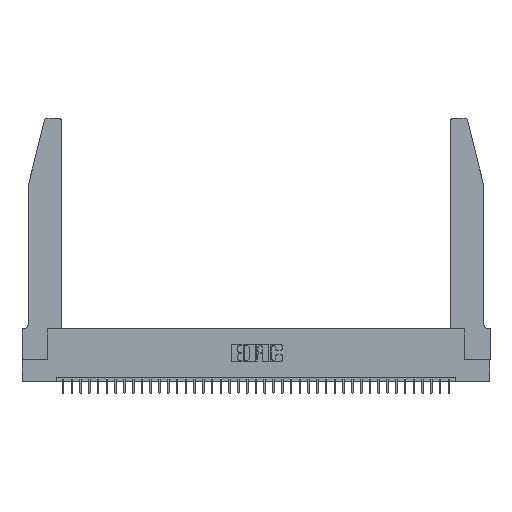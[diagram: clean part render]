
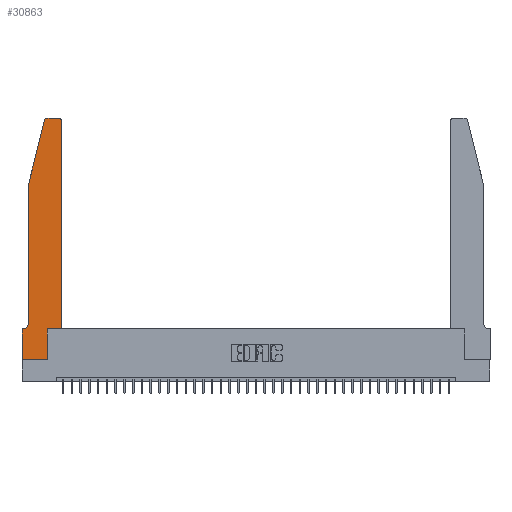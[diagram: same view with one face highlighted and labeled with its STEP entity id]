
A CAD part, top view. The second image highlights one B-rep face of the part: STEP entity #30863.
In plain terms, the highlighted planar face has unit normal (0, 0, 1).
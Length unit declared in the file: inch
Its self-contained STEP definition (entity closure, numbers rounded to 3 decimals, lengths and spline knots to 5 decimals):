
#562 = CARTESIAN_POINT ( 'NONE',  ( 0.0755, 2., 0.37 ) ) ;
#846 = VERTEX_POINT ( 'NONE', #4911 ) ;
#1336 = ORIENTED_EDGE ( 'NONE', *, *, #19822, .T. ) ;
#3396 = CARTESIAN_POINT ( 'NONE',  ( 0.4205, 2.75, 0.37 ) ) ;
#3453 = ORIENTED_EDGE ( 'NONE', *, *, #31086, .T. ) ;
#3972 = AXIS2_PLACEMENT_3D ( 'NONE', #11596, #9017, #30177 ) ;
#4036 = VERTEX_POINT ( 'NONE', #11944 ) ;
#4391 = DIRECTION ( 'NONE',  ( 0., 0., 1. ) ) ;
#4592 = CARTESIAN_POINT ( 'NONE',  ( 0.4505, 0.35, 0.37 ) ) ;
#4911 = CARTESIAN_POINT ( 'NONE',  ( 0.0755, 0.42, 0.37 ) ) ;
#4952 = CARTESIAN_POINT ( 'NONE',  ( 0.4505, 0.35, 0.37 ) ) ;
#5222 = EDGE_LOOP ( 'NONE', ( #11643, #7129, #3453, #20036, #16266, #17601, #38189, #1336, #23816, #18068, #13934, #29057 ) ) ;
#6206 = EDGE_CURVE ( 'NONE', #8929, #23607, #17428, .T. ) ;
#6421 = EDGE_CURVE ( 'NONE', #12799, #4036, #24186, .T. ) ;
#6811 = CIRCLE ( 'NONE', #16441, 0.07 ) ;
#7129 = ORIENTED_EDGE ( 'NONE', *, *, #6421, .T. ) ;
#7367 = DIRECTION ( 'NONE',  ( 0., -1., 0. ) ) ;
#8283 = DIRECTION ( 'NONE',  ( -1., 0., 0. ) ) ;
#8426 = DIRECTION ( 'NONE',  ( -0.239, -0.971, 0. ) ) ;
#8475 = LINE ( 'NONE', #38918, #14270 ) ;
#8929 = VERTEX_POINT ( 'NONE', #26521 ) ;
#9017 = DIRECTION ( 'NONE',  ( 0., 0., 1. ) ) ;
#10393 = CARTESIAN_POINT ( 'NONE',  ( 0.0755, 2., 0.37 ) ) ;
#10853 = VERTEX_POINT ( 'NONE', #15062 ) ;
#11596 = CARTESIAN_POINT ( 'NONE',  ( 0.4205, 2.72, 0.37 ) ) ;
#11643 = ORIENTED_EDGE ( 'NONE', *, *, #32040, .T. ) ;
#11944 = CARTESIAN_POINT ( 'NONE',  ( 0.25487, 2.72718, 0.37 ) ) ;
#12105 = CARTESIAN_POINT ( 'NONE',  ( 0., 0., 0.37 ) ) ;
#12799 = VERTEX_POINT ( 'NONE', #17541 ) ;
#13056 = DIRECTION ( 'NONE',  ( 1., 0., 0. ) ) ;
#13934 = ORIENTED_EDGE ( 'NONE', *, *, #14338, .T. ) ;
#14270 = VECTOR ( 'NONE', #8283, 39.37008 ) ;
#14338 = EDGE_CURVE ( 'NONE', #33840, #8929, #25955, .T. ) ;
#14524 = LINE ( 'NONE', #26473, #16282 ) ;
#14701 = VERTEX_POINT ( 'NONE', #25518 ) ;
#15062 = CARTESIAN_POINT ( 'NONE',  ( 0., 0.35, 0.37 ) ) ;
#15073 = LINE ( 'NONE', #26648, #18429 ) ;
#15681 = DIRECTION ( 'NONE',  ( 0., 0., 1. ) ) ;
#16266 = ORIENTED_EDGE ( 'NONE', *, *, #21156, .T. ) ;
#16282 = VECTOR ( 'NONE', #38733, 39.37008 ) ;
#16441 = AXIS2_PLACEMENT_3D ( 'NONE', #30431, #17532, #39479 ) ;
#16902 = CARTESIAN_POINT ( 'NONE',  ( 0.0055, 0.35, 0.37 ) ) ;
#17428 = CIRCLE ( 'NONE', #3972, 0.03 ) ;
#17532 = DIRECTION ( 'NONE',  ( 0., 0., -1. ) ) ;
#17536 = DIRECTION ( 'NONE',  ( 0., 1., 0. ) ) ;
#17541 = CARTESIAN_POINT ( 'NONE',  ( 0.284, 2.75, 0.37 ) ) ;
#17601 = ORIENTED_EDGE ( 'NONE', *, *, #30661, .T. ) ;
#18068 = ORIENTED_EDGE ( 'NONE', *, *, #31601, .T. ) ;
#18133 = AXIS2_PLACEMENT_3D ( 'NONE', #33867, #15681, #13056 ) ;
#18346 = CARTESIAN_POINT ( 'NONE',  ( 0.2865, 0.35, 0.37 ) ) ;
#18429 = VECTOR ( 'NONE', #26835, 39.37008 ) ;
#18976 = VERTEX_POINT ( 'NONE', #16902 ) ;
#19073 = DIRECTION ( 'NONE',  ( 0., 1., 0. ) ) ;
#19822 = EDGE_CURVE ( 'NONE', #36558, #25336, #21403, .T. ) ;
#20036 = ORIENTED_EDGE ( 'NONE', *, *, #22784, .T. ) ;
#21156 = EDGE_CURVE ( 'NONE', #846, #18976, #6811, .T. ) ;
#21403 = LINE ( 'NONE', #12105, #35076 ) ;
#21962 = FACE_OUTER_BOUND ( 'NONE', #5222, .T. ) ;
#22784 = EDGE_CURVE ( 'NONE', #24928, #846, #31344, .T. ) ;
#23302 = LINE ( 'NONE', #36367, #36253 ) ;
#23509 = DIRECTION ( 'NONE',  ( 1., 0., 0. ) ) ;
#23607 = VERTEX_POINT ( 'NONE', #3396 ) ;
#23816 = ORIENTED_EDGE ( 'NONE', *, *, #38608, .T. ) ;
#24186 = CIRCLE ( 'NONE', #37626, 0.03 ) ;
#24928 = VERTEX_POINT ( 'NONE', #10393 ) ;
#25336 = VERTEX_POINT ( 'NONE', #33922 ) ;
#25518 = CARTESIAN_POINT ( 'NONE',  ( 0.2865, 0.35, 0.37 ) ) ;
#25955 = LINE ( 'NONE', #4592, #39331 ) ;
#26473 = CARTESIAN_POINT ( 'NONE',  ( 0.2605, 2.75, 0.37 ) ) ;
#26521 = CARTESIAN_POINT ( 'NONE',  ( 0.4505, 2.72, 0.37 ) ) ;
#26648 = CARTESIAN_POINT ( 'NONE',  ( 0., 0., 0.37 ) ) ;
#26835 = DIRECTION ( 'NONE',  ( 0., -1., 0. ) ) ;
#28956 = CARTESIAN_POINT ( 'NONE',  ( 0.284, 2.72, 0.37 ) ) ;
#29057 = ORIENTED_EDGE ( 'NONE', *, *, #6206, .T. ) ;
#29632 = CARTESIAN_POINT ( 'NONE',  ( 0.0755, 2., 0.37 ) ) ;
#30177 = DIRECTION ( 'NONE',  ( 1., 0., 0. ) ) ;
#30431 = CARTESIAN_POINT ( 'NONE',  ( 0.0055, 0.42, 0.37 ) ) ;
#30661 = EDGE_CURVE ( 'NONE', #18976, #10853, #8475, .T. ) ;
#30863 = ADVANCED_FACE ( 'NONE', ( #21962 ), #36874, .T. ) ;
#31086 = EDGE_CURVE ( 'NONE', #4036, #24928, #36649, .T. ) ;
#31344 = LINE ( 'NONE', #562, #32025 ) ;
#31560 = CARTESIAN_POINT ( 'NONE',  ( 0., 0., 0.37 ) ) ;
#31601 = EDGE_CURVE ( 'NONE', #14701, #33840, #23302, .T. ) ;
#32025 = VECTOR ( 'NONE', #7367, 39.37008 ) ;
#32040 = EDGE_CURVE ( 'NONE', #23607, #12799, #14524, .T. ) ;
#33277 = VECTOR ( 'NONE', #17536, 39.37008 ) ;
#33674 = LINE ( 'NONE', #18346, #33277 ) ;
#33840 = VERTEX_POINT ( 'NONE', #4952 ) ;
#33867 = CARTESIAN_POINT ( 'NONE',  ( 0., 0.35, 0.37 ) ) ;
#33922 = CARTESIAN_POINT ( 'NONE',  ( 0.2865, 0., 0.37 ) ) ;
#35076 = VECTOR ( 'NONE', #39721, 39.37008 ) ;
#35575 = VECTOR ( 'NONE', #8426, 39.37008 ) ;
#35807 = DIRECTION ( 'NONE',  ( 1., 0., 0. ) ) ;
#36253 = VECTOR ( 'NONE', #23509, 39.37008 ) ;
#36367 = CARTESIAN_POINT ( 'NONE',  ( 0.4505, 0.35, 0.37 ) ) ;
#36558 = VERTEX_POINT ( 'NONE', #31560 ) ;
#36649 = LINE ( 'NONE', #29632, #35575 ) ;
#36874 = PLANE ( 'NONE',  #18133 ) ;
#37496 = EDGE_CURVE ( 'NONE', #10853, #36558, #15073, .T. ) ;
#37626 = AXIS2_PLACEMENT_3D ( 'NONE', #28956, #4391, #35807 ) ;
#38189 = ORIENTED_EDGE ( 'NONE', *, *, #37496, .T. ) ;
#38608 = EDGE_CURVE ( 'NONE', #25336, #14701, #33674, .T. ) ;
#38733 = DIRECTION ( 'NONE',  ( -1., 0., 0. ) ) ;
#38918 = CARTESIAN_POINT ( 'NONE',  ( 0.0755, 0.35, 0.37 ) ) ;
#39331 = VECTOR ( 'NONE', #19073, 39.37008 ) ;
#39479 = DIRECTION ( 'NONE',  ( -1., 0., 0. ) ) ;
#39721 = DIRECTION ( 'NONE',  ( 1., 0., 0. ) ) ;
